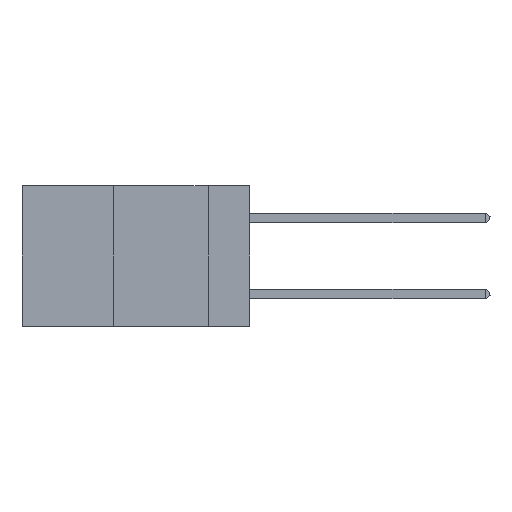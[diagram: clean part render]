
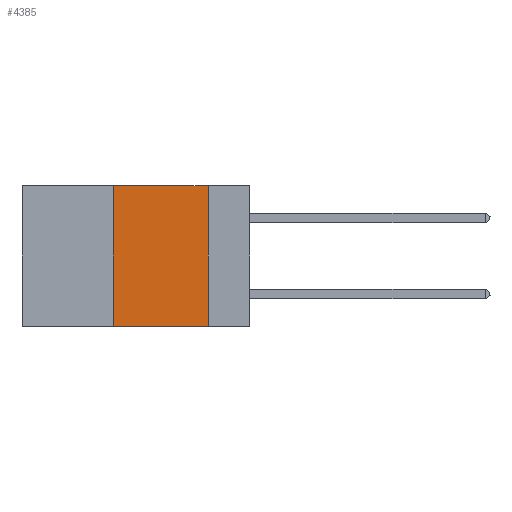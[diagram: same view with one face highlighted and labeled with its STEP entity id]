
A CAD part, left-side view. The second image highlights one B-rep face of the part: STEP entity #4385.
In plain terms, the highlighted planar face has unit normal (-1, 0, 0).
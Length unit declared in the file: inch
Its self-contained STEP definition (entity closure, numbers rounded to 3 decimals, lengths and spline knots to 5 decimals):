
#91 = VERTEX_POINT ( 'NONE', #15408 ) ;
#283 = CARTESIAN_POINT ( 'NONE',  ( 0., 0.6, -0.37 ) ) ;
#1032 = AXIS2_PLACEMENT_3D ( 'NONE', #4571, #16902, #12920 ) ;
#1370 = LINE ( 'NONE', #283, #10473 ) ;
#2247 = DIRECTION ( 'NONE',  ( 0., -1., 0. ) ) ;
#3291 = FACE_OUTER_BOUND ( 'NONE', #19726, .T. ) ;
#3859 = CARTESIAN_POINT ( 'NONE',  ( 0., 0.11, -0.37 ) ) ;
#4058 = DIRECTION ( 'NONE',  ( 0., 0., -1. ) ) ;
#4288 = LINE ( 'NONE', #16435, #17430 ) ;
#4385 = ADVANCED_FACE ( 'NONE', ( #3291 ), #22369, .F. ) ;
#4571 = CARTESIAN_POINT ( 'NONE',  ( 0., 0.6, 0. ) ) ;
#4636 = VECTOR ( 'NONE', #4058, 39.37008 ) ;
#4679 = ORIENTED_EDGE ( 'NONE', *, *, #19021, .F. ) ;
#6987 = CARTESIAN_POINT ( 'NONE',  ( 0., 0.36, -0.37 ) ) ;
#6999 = VECTOR ( 'NONE', #11999, 39.37008 ) ;
#7056 = EDGE_CURVE ( 'NONE', #22144, #11674, #23054, .T. ) ;
#10473 = VECTOR ( 'NONE', #2247, 39.37008 ) ;
#11674 = VERTEX_POINT ( 'NONE', #3859 ) ;
#11754 = EDGE_CURVE ( 'NONE', #13316, #11674, #1370, .T. ) ;
#11999 = DIRECTION ( 'NONE',  ( 0., -1., 0. ) ) ;
#12920 = DIRECTION ( 'NONE',  ( 0., 0., -1. ) ) ;
#13316 = VERTEX_POINT ( 'NONE', #6987 ) ;
#14632 = DIRECTION ( 'NONE',  ( 0., 0., 1. ) ) ;
#14706 = ORIENTED_EDGE ( 'NONE', *, *, #11754, .T. ) ;
#14761 = CARTESIAN_POINT ( 'NONE',  ( 0., 0.11, 0. ) ) ;
#15098 = ORIENTED_EDGE ( 'NONE', *, *, #7056, .F. ) ;
#15408 = CARTESIAN_POINT ( 'NONE',  ( 0., 0.36, 0. ) ) ;
#16218 = EDGE_CURVE ( 'NONE', #13316, #91, #4288, .T. ) ;
#16435 = CARTESIAN_POINT ( 'NONE',  ( 0., 0.36, 0. ) ) ;
#16902 = DIRECTION ( 'NONE',  ( 1., 0., 0. ) ) ;
#17240 = CARTESIAN_POINT ( 'NONE',  ( 0., 0.11, 0. ) ) ;
#17430 = VECTOR ( 'NONE', #14632, 39.37008 ) ;
#18217 = ORIENTED_EDGE ( 'NONE', *, *, #16218, .F. ) ;
#19021 = EDGE_CURVE ( 'NONE', #91, #22144, #21199, .T. ) ;
#19083 = CARTESIAN_POINT ( 'NONE',  ( 0., 0.6, 0. ) ) ;
#19726 = EDGE_LOOP ( 'NONE', ( #15098, #4679, #18217, #14706 ) ) ;
#21199 = LINE ( 'NONE', #19083, #6999 ) ;
#22144 = VERTEX_POINT ( 'NONE', #17240 ) ;
#22369 = PLANE ( 'NONE',  #1032 ) ;
#23054 = LINE ( 'NONE', #14761, #4636 ) ;
